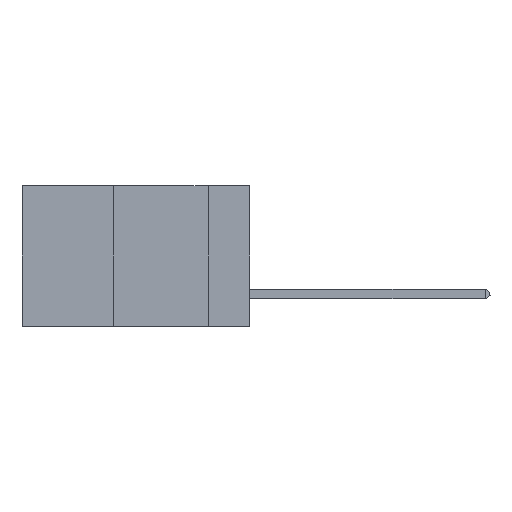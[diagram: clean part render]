
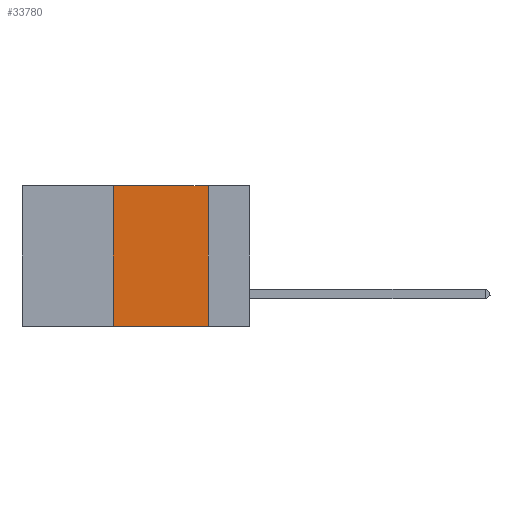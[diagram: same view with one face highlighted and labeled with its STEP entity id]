
A CAD part, left-side view. The second image highlights one B-rep face of the part: STEP entity #33780.
In plain terms, the highlighted planar face has unit normal (-1, 0, 0).
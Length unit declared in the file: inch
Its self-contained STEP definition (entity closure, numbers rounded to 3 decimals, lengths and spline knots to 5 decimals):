
#1280 = ORIENTED_EDGE ( 'NONE', *, *, #29861, .T. ) ;
#1361 = DIRECTION ( 'NONE',  ( 1., 0., 0. ) ) ;
#2190 = DIRECTION ( 'NONE',  ( 0., -1., 0. ) ) ;
#3121 = EDGE_LOOP ( 'NONE', ( #22303, #16015, #29784, #1280 ) ) ;
#4419 = DIRECTION ( 'NONE',  ( 0., 0., -1. ) ) ;
#5460 = CARTESIAN_POINT ( 'NONE',  ( 0., 0.6, 0. ) ) ;
#6296 = FACE_OUTER_BOUND ( 'NONE', #3121, .T. ) ;
#8037 = EDGE_CURVE ( 'NONE', #25194, #14508, #29025, .T. ) ;
#11215 = DIRECTION ( 'NONE',  ( 0., 0., -1. ) ) ;
#11303 = VECTOR ( 'NONE', #2190, 39.37008 ) ;
#11633 = VECTOR ( 'NONE', #42632, 39.37008 ) ;
#13892 = CARTESIAN_POINT ( 'NONE',  ( 0., 0.11, 0. ) ) ;
#14508 = VERTEX_POINT ( 'NONE', #13892 ) ;
#16015 = ORIENTED_EDGE ( 'NONE', *, *, #8037, .F. ) ;
#18159 = LINE ( 'NONE', #22273, #11303 ) ;
#21068 = CARTESIAN_POINT ( 'NONE',  ( 0., 0.11, -0.37 ) ) ;
#21584 = PLANE ( 'NONE',  #30666 ) ;
#22031 = DIRECTION ( 'NONE',  ( 0., 0., 1. ) ) ;
#22273 = CARTESIAN_POINT ( 'NONE',  ( 0., 0.6, -0.37 ) ) ;
#22303 = ORIENTED_EDGE ( 'NONE', *, *, #42446, .F. ) ;
#24178 = CARTESIAN_POINT ( 'NONE',  ( 0., 0.11, 0. ) ) ;
#24357 = CARTESIAN_POINT ( 'NONE',  ( 0., 0.36, -0.37 ) ) ;
#24989 = LINE ( 'NONE', #24178, #39672 ) ;
#25095 = CARTESIAN_POINT ( 'NONE',  ( 0., 0.6, 0. ) ) ;
#25194 = VERTEX_POINT ( 'NONE', #28030 ) ;
#28030 = CARTESIAN_POINT ( 'NONE',  ( 0., 0.36, 0. ) ) ;
#28546 = EDGE_CURVE ( 'NONE', #40255, #25194, #30416, .T. ) ;
#29025 = LINE ( 'NONE', #5460, #11633 ) ;
#29784 = ORIENTED_EDGE ( 'NONE', *, *, #28546, .F. ) ;
#29861 = EDGE_CURVE ( 'NONE', #40255, #35694, #18159, .T. ) ;
#30416 = LINE ( 'NONE', #38410, #38241 ) ;
#30666 = AXIS2_PLACEMENT_3D ( 'NONE', #25095, #1361, #11215 ) ;
#33780 = ADVANCED_FACE ( 'NONE', ( #6296 ), #21584, .F. ) ;
#35694 = VERTEX_POINT ( 'NONE', #21068 ) ;
#38241 = VECTOR ( 'NONE', #22031, 39.37008 ) ;
#38410 = CARTESIAN_POINT ( 'NONE',  ( 0., 0.36, 0. ) ) ;
#39672 = VECTOR ( 'NONE', #4419, 39.37008 ) ;
#40255 = VERTEX_POINT ( 'NONE', #24357 ) ;
#42446 = EDGE_CURVE ( 'NONE', #14508, #35694, #24989, .T. ) ;
#42632 = DIRECTION ( 'NONE',  ( 0., -1., 0. ) ) ;
